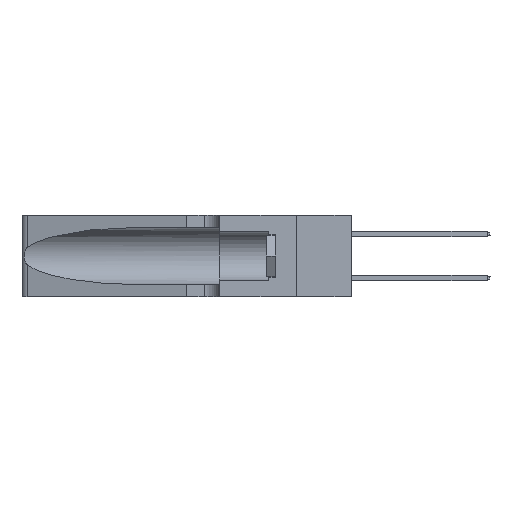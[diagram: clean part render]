
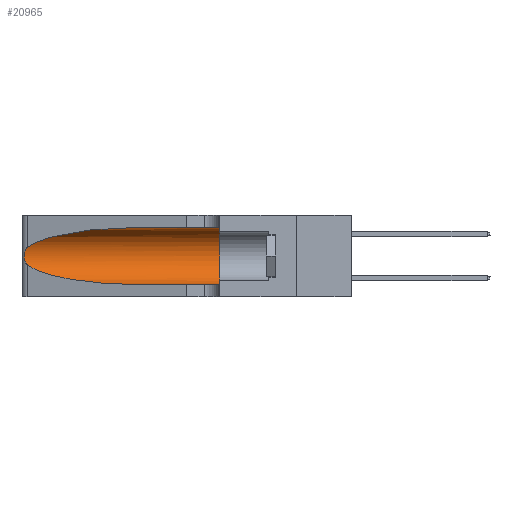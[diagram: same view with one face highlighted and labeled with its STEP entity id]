
A CAD part, left-side view. The second image highlights one B-rep face of the part: STEP entity #20965.
In plain terms, the highlighted cylindrical face has radius 3.308 mm (diameter 6.617 mm), a partial arc.
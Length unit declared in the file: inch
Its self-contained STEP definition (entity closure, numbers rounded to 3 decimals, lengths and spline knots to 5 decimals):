
#163 = ORIENTED_EDGE ( 'NONE', *, *, #13188, .F. ) ;
#544 = CARTESIAN_POINT ( 'NONE',  ( 0.25555, 1.22993, 0.14849 ) ) ;
#722 = EDGE_CURVE ( 'NONE', #16499, #18349, #18773, .T. ) ;
#757 = LINE ( 'NONE', #2587, #10561 ) ;
#769 = B_SPLINE_CURVE_WITH_KNOTS ( 'NONE', 3,
 ( #15149, #13356, #6046, #4253, #16934, #6124, #18680, #7978, #20452, #9774, #22200, #11611, #544, #13429 ),
 .UNSPECIFIED., .F., .F.,
 ( 4, 2, 2, 2, 2, 2, 4 ),
 ( 0., 0.00027, 0.00053, 0.00107, 0.0016, 0.00187, 0.00214 ),
 .UNSPECIFIED. ) ;
#2587 = CARTESIAN_POINT ( 'NONE',  ( 0.1305, 1.61858, 0.05475 ) ) ;
#2730 = CARTESIAN_POINT ( 'NONE',  ( 0.1305, 1.61858, 0.185 ) ) ;
#4227 = CARTESIAN_POINT ( 'NONE',  ( 0.2373, 1.15595, 0.08982 ) ) ;
#4253 = CARTESIAN_POINT ( 'NONE',  ( 0.25787, 1.23484, 0.2124 ) ) ;
#4484 = EDGE_CURVE ( 'NONE', #22706, #21330, #769, .T. ) ;
#5096 = CARTESIAN_POINT ( 'NONE',  ( 0.1305, 1.61858, 0.31525 ) ) ;
#5425 = CARTESIAN_POINT ( 'NONE',  ( 0.18966, 0.96281, 0.31525 ) ) ;
#5587 = CARTESIAN_POINT ( 'NONE',  ( 0.25487, 1.22718, 0.22369 ) ) ;
#5827 = ORIENTED_EDGE ( 'NONE', *, *, #4484, .T. ) ;
#6046 = CARTESIAN_POINT ( 'NONE',  ( 0.25639, 1.23184, 0.21858 ) ) ;
#6075 = CARTESIAN_POINT ( 'NONE',  ( 0.1305, 0.35, 0.31525 ) ) ;
#6090 = CARTESIAN_POINT ( 'NONE',  ( 0.18966, 0.96281, 0.05475 ) ) ;
#6124 = CARTESIAN_POINT ( 'NONE',  ( 0.26018, 1.23835, 0.19895 ) ) ;
#6464 = DIRECTION ( 'NONE',  ( 0., -1., 0. ) ) ;
#7978 = CARTESIAN_POINT ( 'NONE',  ( 0.26075, 1.23896, 0.178 ) ) ;
#8367 =( BOUNDED_CURVE ( )  B_SPLINE_CURVE ( 3, ( #19857, #5425, #16429, #5587 ),
 .UNSPECIFIED., .F., .T. ) 
 B_SPLINE_CURVE_WITH_KNOTS ( ( 4, 4 ),
 ( 1.5708, 2.84003 ),
 .UNSPECIFIED. ) 
 CURVE ( )  GEOMETRIC_REPRESENTATION_ITEM ( )  RATIONAL_B_SPLINE_CURVE ( ( 1., 0.87, 0.87, 1. ) ) 
 REPRESENTATION_ITEM ( '' )  );
#8831 = CARTESIAN_POINT ( 'NONE',  ( 0.1305, 0.35, 0.185 ) ) ;
#9292 = CARTESIAN_POINT ( 'NONE',  ( 0.25487, 1.22718, 0.14631 ) ) ;
#9418 = EDGE_CURVE ( 'NONE', #17606, #13095, #757, .T. ) ;
#9477 = ORIENTED_EDGE ( 'NONE', *, *, #722, .F. ) ;
#9540 = ORIENTED_EDGE ( 'NONE', *, *, #9418, .T. ) ;
#9774 = CARTESIAN_POINT ( 'NONE',  ( 0.25856, 1.23593, 0.16098 ) ) ;
#9947 = DIRECTION ( 'NONE',  ( 0., -1., 0. ) ) ;
#10561 = VECTOR ( 'NONE', #9947, 39.37008 ) ;
#10631 = DIRECTION ( 'NONE',  ( 0., 0., 1. ) ) ;
#10816 =( BOUNDED_CURVE ( )  B_SPLINE_CURVE ( 3, ( #15118, #4227, #6090, #18643 ),
 .UNSPECIFIED., .F., .T. ) 
 B_SPLINE_CURVE_WITH_KNOTS ( ( 4, 4 ),
 ( 3.44316, 4.71239 ),
 .UNSPECIFIED. ) 
 CURVE ( )  GEOMETRIC_REPRESENTATION_ITEM ( )  RATIONAL_B_SPLINE_CURVE ( ( 1., 0.87, 0.87, 1. ) ) 
 REPRESENTATION_ITEM ( '' )  );
#11456 = CARTESIAN_POINT ( 'NONE',  ( 0.25487, 1.22718, 0.22369 ) ) ;
#11611 = CARTESIAN_POINT ( 'NONE',  ( 0.25639, 1.23186, 0.15144 ) ) ;
#11921 = DIRECTION ( 'NONE',  ( 0., -1., 0. ) ) ;
#12724 = AXIS2_PLACEMENT_3D ( 'NONE', #2730, #11921, #22503 ) ;
#13095 = VERTEX_POINT ( 'NONE', #22730 ) ;
#13188 = EDGE_CURVE ( 'NONE', #18349, #13095, #18938, .T. ) ;
#13356 = CARTESIAN_POINT ( 'NONE',  ( 0.25555, 1.22994, 0.2215 ) ) ;
#13429 = CARTESIAN_POINT ( 'NONE',  ( 0.25487, 1.22718, 0.14631 ) ) ;
#13638 = CYLINDRICAL_SURFACE ( 'NONE', #12724, 0.13025 ) ;
#13979 = EDGE_CURVE ( 'NONE', #16499, #22706, #8367, .T. ) ;
#14171 = CARTESIAN_POINT ( 'NONE',  ( 0.1305, 0.72297, 0.31525 ) ) ;
#14341 = ORIENTED_EDGE ( 'NONE', *, *, #21507, .T. ) ;
#15118 = CARTESIAN_POINT ( 'NONE',  ( 0.25487, 1.22718, 0.14631 ) ) ;
#15149 = CARTESIAN_POINT ( 'NONE',  ( 0.25487, 1.22718, 0.22369 ) ) ;
#15992 = EDGE_LOOP ( 'NONE', ( #16010, #5827, #14341, #9540, #163, #9477 ) ) ;
#16010 = ORIENTED_EDGE ( 'NONE', *, *, #13979, .T. ) ;
#16429 = CARTESIAN_POINT ( 'NONE',  ( 0.2373, 1.15595, 0.28018 ) ) ;
#16499 = VERTEX_POINT ( 'NONE', #14171 ) ;
#16934 = CARTESIAN_POINT ( 'NONE',  ( 0.25854, 1.2359, 0.20912 ) ) ;
#17541 = AXIS2_PLACEMENT_3D ( 'NONE', #8831, #21253, #10631 ) ;
#17606 = VERTEX_POINT ( 'NONE', #22352 ) ;
#18349 = VERTEX_POINT ( 'NONE', #6075 ) ;
#18643 = CARTESIAN_POINT ( 'NONE',  ( 0.1305, 0.72297, 0.05475 ) ) ;
#18680 = CARTESIAN_POINT ( 'NONE',  ( 0.26075, 1.23896, 0.19203 ) ) ;
#18773 = LINE ( 'NONE', #5096, #19305 ) ;
#18938 = CIRCLE ( 'NONE', #17541, 0.13025 ) ;
#19305 = VECTOR ( 'NONE', #6464, 39.37008 ) ;
#19857 = CARTESIAN_POINT ( 'NONE',  ( 0.1305, 0.72297, 0.31525 ) ) ;
#20452 = CARTESIAN_POINT ( 'NONE',  ( 0.26017, 1.23833, 0.17102 ) ) ;
#20965 = ADVANCED_FACE ( 'NONE', ( #22987 ), #13638, .F. ) ;
#21253 = DIRECTION ( 'NONE',  ( 0., 1., 0. ) ) ;
#21330 = VERTEX_POINT ( 'NONE', #9292 ) ;
#21507 = EDGE_CURVE ( 'NONE', #21330, #17606, #10816, .T. ) ;
#22200 = CARTESIAN_POINT ( 'NONE',  ( 0.25789, 1.23486, 0.15765 ) ) ;
#22352 = CARTESIAN_POINT ( 'NONE',  ( 0.1305, 0.72297, 0.05475 ) ) ;
#22503 = DIRECTION ( 'NONE',  ( 0., 0., -1. ) ) ;
#22706 = VERTEX_POINT ( 'NONE', #11456 ) ;
#22730 = CARTESIAN_POINT ( 'NONE',  ( 0.1305, 0.35, 0.05475 ) ) ;
#22987 = FACE_OUTER_BOUND ( 'NONE', #15992, .T. ) ;
